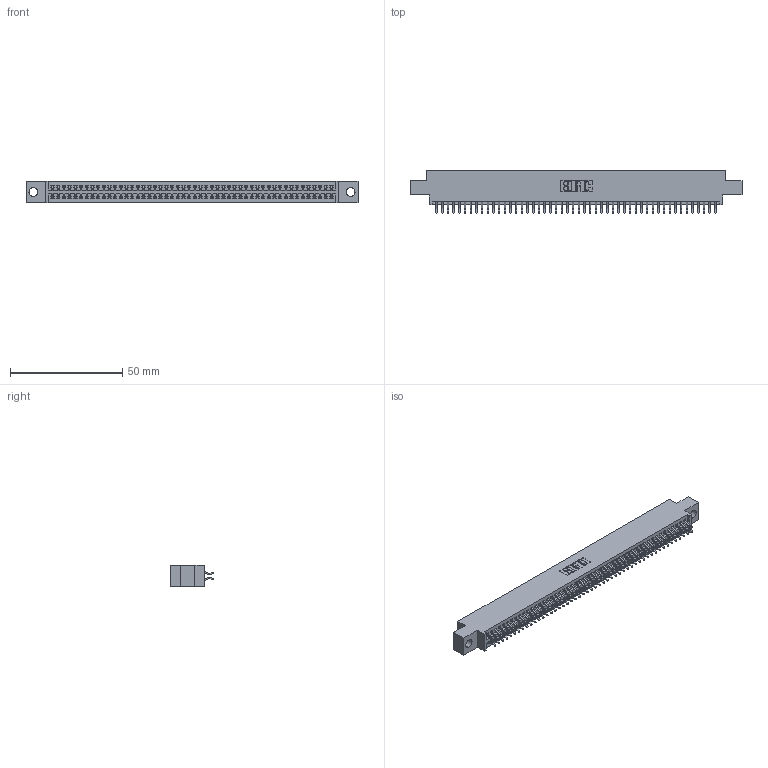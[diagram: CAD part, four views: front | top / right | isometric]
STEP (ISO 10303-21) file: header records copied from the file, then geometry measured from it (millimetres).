
FILE_DESCRIPTION (( 'STEP AP203' ), '1' );
FILE_NAME ('345-100-556-804.STEP', '2021-05-20T19:05:33', ( '' ), ( '' ), 'SwSTEP 2.0', 'SolidWorks 2020', '' );
FILE_SCHEMA (( 'CONFIG_CONTROL_DESIGN' ));
Length unit declared in the file: inch
Products named in the file (3): 345-100-556-804; 345-292-001_556 Tail; 345 Part_0.170 Offset - 0.156 Dia-TI
Assembly tree (101 placements, depth 2):
  345-100-556-804
    345 Part_0.170 Offset - 0.156 Dia-TI
    345-292-001_556 Tail  x100
Bounding box: 148.21 x 19.24 x 9.4 mm (x, y, z)
Volume: 14248.1 mm3; surface area: 21123.6 mm2
Topology: 101 solids, 101 shells, 5744 faces, 17089 edges, 11258 vertices
Faces by surface type: plane 3798, cylinder 1946
Entity records: 38925 total; most frequent: CARTESIAN_POINT 6538, ORIENTED_EDGE 6458, DIRECTION 5741, EDGE_CURVE 3229, VECTOR 2889, LINE 2889, VERTEX_POINT 2150, AXIS2_PLACEMENT_3D 1426
